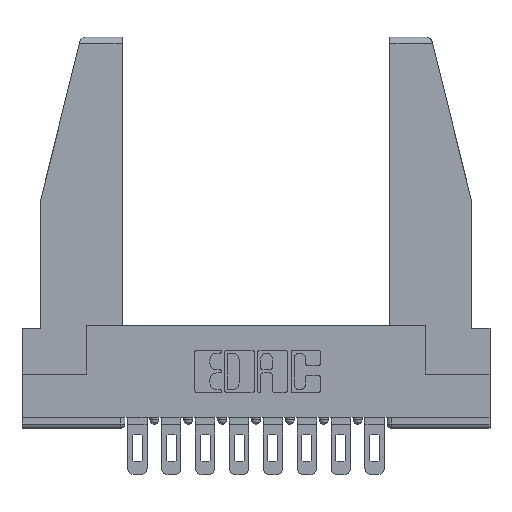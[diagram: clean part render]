
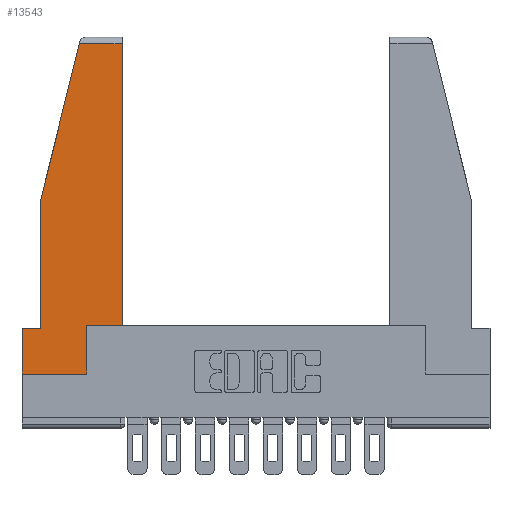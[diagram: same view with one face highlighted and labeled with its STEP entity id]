
A CAD part, top view. The second image highlights one B-rep face of the part: STEP entity #13543.
In plain terms, the highlighted planar face has unit normal (0, 0, 1).
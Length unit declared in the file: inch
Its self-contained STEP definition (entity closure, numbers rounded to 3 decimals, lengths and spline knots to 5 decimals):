
#91 = LINE ( 'NONE', #10045, #5803 ) ;
#240 = CARTESIAN_POINT ( 'NONE',  ( 0.086, 0.21, 0. ) ) ;
#302 = DIRECTION ( 'NONE',  ( -0.239, -0.971, 0. ) ) ;
#379 = ORIENTED_EDGE ( 'NONE', *, *, #7894, .T. ) ;
#639 = DIRECTION ( 'NONE',  ( -1., 0., 0. ) ) ;
#678 = VERTEX_POINT ( 'NONE', #9674 ) ;
#746 = EDGE_CURVE ( 'NONE', #678, #3564, #8597, .T. ) ;
#920 = EDGE_CURVE ( 'NONE', #3564, #6166, #7997, .T. ) ;
#1164 = VECTOR ( 'NONE', #11091, 39.37008 ) ;
#1395 = CARTESIAN_POINT ( 'NONE',  ( 0.297, 0.223, 0. ) ) ;
#1487 = DIRECTION ( 'NONE',  ( 1., 0., 0. ) ) ;
#1932 = CARTESIAN_POINT ( 'NONE',  ( 0.086, 0.8, 0. ) ) ;
#2118 = ORIENTED_EDGE ( 'NONE', *, *, #920, .T. ) ;
#2274 = CARTESIAN_POINT ( 'NONE',  ( 0., 0.21, 0. ) ) ;
#2651 = VECTOR ( 'NONE', #8178, 39.37008 ) ;
#2660 = VECTOR ( 'NONE', #639, 39.37008 ) ;
#3544 = ORIENTED_EDGE ( 'NONE', *, *, #10479, .T. ) ;
#3564 = VERTEX_POINT ( 'NONE', #240 ) ;
#3816 = LINE ( 'NONE', #9105, #2651 ) ;
#3987 = EDGE_CURVE ( 'NONE', #9375, #678, #91, .T. ) ;
#4312 = LINE ( 'NONE', #5415, #1164 ) ;
#4320 = CARTESIAN_POINT ( 'NONE',  ( 0.461, 1.52, 0. ) ) ;
#4728 = LINE ( 'NONE', #11575, #12064 ) ;
#4841 = AXIS2_PLACEMENT_3D ( 'NONE', #13670, #5934, #1487 ) ;
#5397 = ORIENTED_EDGE ( 'NONE', *, *, #10338, .T. ) ;
#5415 = CARTESIAN_POINT ( 'NONE',  ( 0.297, 0., 0. ) ) ;
#5650 = CARTESIAN_POINT ( 'NONE',  ( 0.297, 0., 0. ) ) ;
#5753 = VERTEX_POINT ( 'NONE', #8960 ) ;
#5762 = LINE ( 'NONE', #1395, #9965 ) ;
#5803 = VECTOR ( 'NONE', #302, 39.37008 ) ;
#5911 = ORIENTED_EDGE ( 'NONE', *, *, #7031, .T. ) ;
#5934 = DIRECTION ( 'NONE',  ( 0., 0., 1. ) ) ;
#6166 = VERTEX_POINT ( 'NONE', #2274 ) ;
#6271 = VECTOR ( 'NONE', #12071, 39.37008 ) ;
#6312 = CARTESIAN_POINT ( 'NONE',  ( 0., 1.52, 0. ) ) ;
#6725 = EDGE_LOOP ( 'NONE', ( #7143, #10544, #7037, #7178, #2118, #379, #5911, #5397, #3544 ) ) ;
#7031 = EDGE_CURVE ( 'NONE', #5753, #11000, #3816, .T. ) ;
#7037 = ORIENTED_EDGE ( 'NONE', *, *, #3987, .T. ) ;
#7117 = EDGE_CURVE ( 'NONE', #7388, #9375, #10535, .T. ) ;
#7143 = ORIENTED_EDGE ( 'NONE', *, *, #8165, .T. ) ;
#7178 = ORIENTED_EDGE ( 'NONE', *, *, #746, .T. ) ;
#7388 = VERTEX_POINT ( 'NONE', #4320 ) ;
#7894 = EDGE_CURVE ( 'NONE', #6166, #5753, #4728, .T. ) ;
#7895 = LINE ( 'NONE', #10915, #6271 ) ;
#7936 = DIRECTION ( 'NONE',  ( -1., 0., 0. ) ) ;
#7997 = LINE ( 'NONE', #13505, #12133 ) ;
#8165 = EDGE_CURVE ( 'NONE', #8891, #7388, #7895, .T. ) ;
#8178 = DIRECTION ( 'NONE',  ( 1., 0., 0. ) ) ;
#8597 = LINE ( 'NONE', #1932, #12346 ) ;
#8891 = VERTEX_POINT ( 'NONE', #13942 ) ;
#8960 = CARTESIAN_POINT ( 'NONE',  ( 0., 0., 0. ) ) ;
#9105 = CARTESIAN_POINT ( 'NONE',  ( 0., 0., 0. ) ) ;
#9338 = DIRECTION ( 'NONE',  ( 0., -1., 0. ) ) ;
#9375 = VERTEX_POINT ( 'NONE', #13041 ) ;
#9674 = CARTESIAN_POINT ( 'NONE',  ( 0.086, 0.8, 0. ) ) ;
#9783 = VERTEX_POINT ( 'NONE', #14036 ) ;
#9965 = VECTOR ( 'NONE', #10157, 39.37008 ) ;
#10045 = CARTESIAN_POINT ( 'NONE',  ( 0.271, 1.55, 0. ) ) ;
#10157 = DIRECTION ( 'NONE',  ( 1., 0., 0. ) ) ;
#10338 = EDGE_CURVE ( 'NONE', #11000, #9783, #4312, .T. ) ;
#10479 = EDGE_CURVE ( 'NONE', #9783, #8891, #5762, .T. ) ;
#10535 = LINE ( 'NONE', #6312, #2660 ) ;
#10544 = ORIENTED_EDGE ( 'NONE', *, *, #7117, .T. ) ;
#10613 = PLANE ( 'NONE',  #4841 ) ;
#10915 = CARTESIAN_POINT ( 'NONE',  ( 0.461, 0.223, 0. ) ) ;
#11000 = VERTEX_POINT ( 'NONE', #5650 ) ;
#11091 = DIRECTION ( 'NONE',  ( 0., 1., 0. ) ) ;
#11575 = CARTESIAN_POINT ( 'NONE',  ( 0., 0.21, 0. ) ) ;
#11627 = FACE_OUTER_BOUND ( 'NONE', #6725, .T. ) ;
#12064 = VECTOR ( 'NONE', #9338, 39.37008 ) ;
#12071 = DIRECTION ( 'NONE',  ( 0., 1., 0. ) ) ;
#12133 = VECTOR ( 'NONE', #7936, 39.37008 ) ;
#12346 = VECTOR ( 'NONE', #13951, 39.37008 ) ;
#13041 = CARTESIAN_POINT ( 'NONE',  ( 0.2636, 1.52, 0. ) ) ;
#13505 = CARTESIAN_POINT ( 'NONE',  ( 0., 0.21, 0. ) ) ;
#13543 = ADVANCED_FACE ( 'NONE', ( #11627 ), #10613, .T. ) ;
#13670 = CARTESIAN_POINT ( 'NONE',  ( 0., 0., 0. ) ) ;
#13942 = CARTESIAN_POINT ( 'NONE',  ( 0.461, 0.223, 0. ) ) ;
#13951 = DIRECTION ( 'NONE',  ( 0., -1., 0. ) ) ;
#14036 = CARTESIAN_POINT ( 'NONE',  ( 0.297, 0.223, 0. ) ) ;
